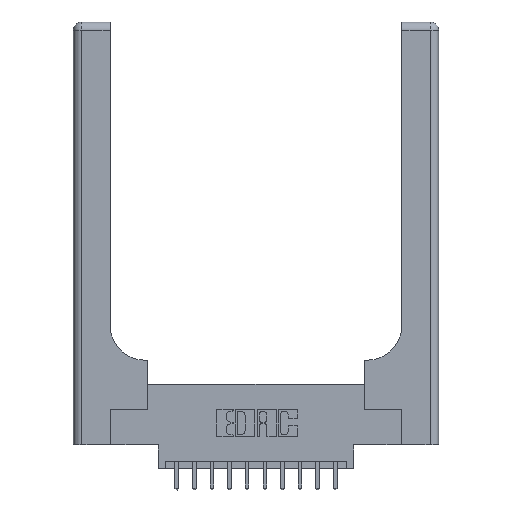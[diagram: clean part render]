
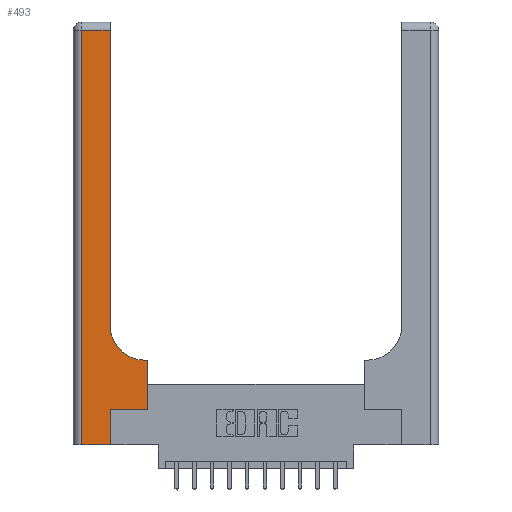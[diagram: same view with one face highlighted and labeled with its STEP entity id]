
A CAD part, top view. The second image highlights one B-rep face of the part: STEP entity #493.
In plain terms, the highlighted planar face has unit normal (0, 0, 1).
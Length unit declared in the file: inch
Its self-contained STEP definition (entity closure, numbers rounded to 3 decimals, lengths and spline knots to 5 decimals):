
#70 = EDGE_CURVE ( 'NONE', #11800, #2465, #2127, .T. ) ;
#493 = ADVANCED_FACE ( 'NONE', ( #9997 ), #6776, .F. ) ;
#584 = VECTOR ( 'NONE', #11333, 39.37008 ) ;
#614 = CARTESIAN_POINT ( 'NONE',  ( 0.528, 0.6, 0.37 ) ) ;
#722 = VERTEX_POINT ( 'NONE', #3367 ) ;
#959 = CARTESIAN_POINT ( 'NONE',  ( 0.528, 0.25, 0.37 ) ) ;
#1030 = CARTESIAN_POINT ( 'NONE',  ( 0.265, 0.25, 0.37 ) ) ;
#1088 = ORIENTED_EDGE ( 'NONE', *, *, #1621, .T. ) ;
#1098 = LINE ( 'NONE', #5391, #14004 ) ;
#1270 = ORIENTED_EDGE ( 'NONE', *, *, #7620, .T. ) ;
#1462 = LINE ( 'NONE', #5951, #13966 ) ;
#1543 = VERTEX_POINT ( 'NONE', #10244 ) ;
#1621 = EDGE_CURVE ( 'NONE', #11309, #13130, #9967, .T. ) ;
#1897 = ORIENTED_EDGE ( 'NONE', *, *, #7758, .T. ) ;
#1982 = CARTESIAN_POINT ( 'NONE',  ( 0.51, 0.85, 0.37 ) ) ;
#2061 = ORIENTED_EDGE ( 'NONE', *, *, #6742, .T. ) ;
#2127 = LINE ( 'NONE', #11487, #14973 ) ;
#2286 = DIRECTION ( 'NONE',  ( 1., 0., 0. ) ) ;
#2465 = VERTEX_POINT ( 'NONE', #614 ) ;
#2893 = VECTOR ( 'NONE', #8912, 39.37008 ) ;
#3091 = ORIENTED_EDGE ( 'NONE', *, *, #70, .T. ) ;
#3259 = DIRECTION ( 'NONE',  ( 1., 0., 0. ) ) ;
#3367 = CARTESIAN_POINT ( 'NONE',  ( 0.06, 0., 0.37 ) ) ;
#4104 = EDGE_CURVE ( 'NONE', #9022, #11800, #9276, .T. ) ;
#4415 = LINE ( 'NONE', #5224, #584 ) ;
#4445 = ORIENTED_EDGE ( 'NONE', *, *, #8470, .T. ) ;
#4705 = ORIENTED_EDGE ( 'NONE', *, *, #4104, .T. ) ;
#5051 = AXIS2_PLACEMENT_3D ( 'NONE', #8155, #9582, #10628 ) ;
#5224 = CARTESIAN_POINT ( 'NONE',  ( 0.26, 3., 0.37 ) ) ;
#5391 = CARTESIAN_POINT ( 'NONE',  ( 0.06, 3., 0.37 ) ) ;
#5951 = CARTESIAN_POINT ( 'NONE',  ( 0.265, 0., 0.37 ) ) ;
#6742 = EDGE_CURVE ( 'NONE', #13130, #722, #1098, .T. ) ;
#6776 = PLANE ( 'NONE',  #5051 ) ;
#7284 = CIRCLE ( 'NONE', #12429, 0.25 ) ;
#7473 = DIRECTION ( 'NONE',  ( 1., 0., 0. ) ) ;
#7507 = VERTEX_POINT ( 'NONE', #9492 ) ;
#7620 = EDGE_CURVE ( 'NONE', #1543, #9022, #1462, .T. ) ;
#7758 = EDGE_CURVE ( 'NONE', #722, #1543, #15697, .T. ) ;
#8155 = CARTESIAN_POINT ( 'NONE',  ( 0., 3., 0.37 ) ) ;
#8414 = VECTOR ( 'NONE', #7473, 39.37008 ) ;
#8470 = EDGE_CURVE ( 'NONE', #2465, #11439, #11794, .T. ) ;
#8587 = VECTOR ( 'NONE', #11228, 39.37008 ) ;
#8912 = DIRECTION ( 'NONE',  ( -1., 0., 0. ) ) ;
#9022 = VERTEX_POINT ( 'NONE', #1030 ) ;
#9205 = CARTESIAN_POINT ( 'NONE',  ( 0., 2.94, 0.37 ) ) ;
#9276 = LINE ( 'NONE', #11025, #12107 ) ;
#9492 = CARTESIAN_POINT ( 'NONE',  ( 0.26, 0.85, 0.37 ) ) ;
#9519 = EDGE_CURVE ( 'NONE', #7507, #11309, #4415, .T. ) ;
#9582 = DIRECTION ( 'NONE',  ( 0., 0., -1. ) ) ;
#9967 = LINE ( 'NONE', #9205, #2893 ) ;
#9997 = FACE_OUTER_BOUND ( 'NONE', #15982, .T. ) ;
#10244 = CARTESIAN_POINT ( 'NONE',  ( 0.265, 0., 0.37 ) ) ;
#10628 = DIRECTION ( 'NONE',  ( -1., 0., 0. ) ) ;
#10768 = DIRECTION ( 'NONE',  ( 0., 0., -1. ) ) ;
#11025 = CARTESIAN_POINT ( 'NONE',  ( 0.265, 0.25, 0.37 ) ) ;
#11044 = CARTESIAN_POINT ( 'NONE',  ( 0., 0., 0.37 ) ) ;
#11228 = DIRECTION ( 'NONE',  ( -1., 0., 0. ) ) ;
#11279 = CARTESIAN_POINT ( 'NONE',  ( 0.26, 2.94, 0.37 ) ) ;
#11301 = DIRECTION ( 'NONE',  ( 0., 1., 0. ) ) ;
#11309 = VERTEX_POINT ( 'NONE', #11279 ) ;
#11333 = DIRECTION ( 'NONE',  ( 0., 1., 0. ) ) ;
#11439 = VERTEX_POINT ( 'NONE', #15274 ) ;
#11487 = CARTESIAN_POINT ( 'NONE',  ( 0.528, 0.25, 0.37 ) ) ;
#11651 = EDGE_CURVE ( 'NONE', #11439, #7507, #7284, .T. ) ;
#11794 = LINE ( 'NONE', #12423, #8587 ) ;
#11800 = VERTEX_POINT ( 'NONE', #959 ) ;
#12107 = VECTOR ( 'NONE', #2286, 39.37008 ) ;
#12124 = DIRECTION ( 'NONE',  ( 0., 1., 0. ) ) ;
#12423 = CARTESIAN_POINT ( 'NONE',  ( 0.26, 0.6, 0.37 ) ) ;
#12429 = AXIS2_PLACEMENT_3D ( 'NONE', #1982, #10768, #3259 ) ;
#12745 = DIRECTION ( 'NONE',  ( 0., -1., 0. ) ) ;
#13130 = VERTEX_POINT ( 'NONE', #13140 ) ;
#13140 = CARTESIAN_POINT ( 'NONE',  ( 0.06, 2.94, 0.37 ) ) ;
#13757 = ORIENTED_EDGE ( 'NONE', *, *, #11651, .T. ) ;
#13966 = VECTOR ( 'NONE', #12124, 39.37008 ) ;
#14004 = VECTOR ( 'NONE', #12745, 39.37008 ) ;
#14973 = VECTOR ( 'NONE', #11301, 39.37008 ) ;
#15274 = CARTESIAN_POINT ( 'NONE',  ( 0.51, 0.6, 0.37 ) ) ;
#15697 = LINE ( 'NONE', #11044, #8414 ) ;
#15982 = EDGE_LOOP ( 'NONE', ( #16005, #1088, #2061, #1897, #1270, #4705, #3091, #4445, #13757 ) ) ;
#16005 = ORIENTED_EDGE ( 'NONE', *, *, #9519, .T. ) ;
